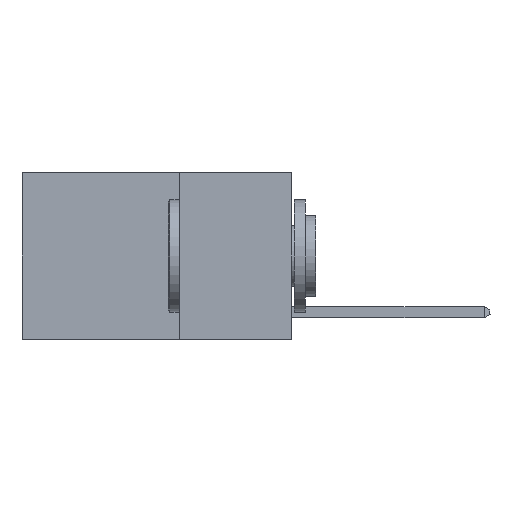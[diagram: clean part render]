
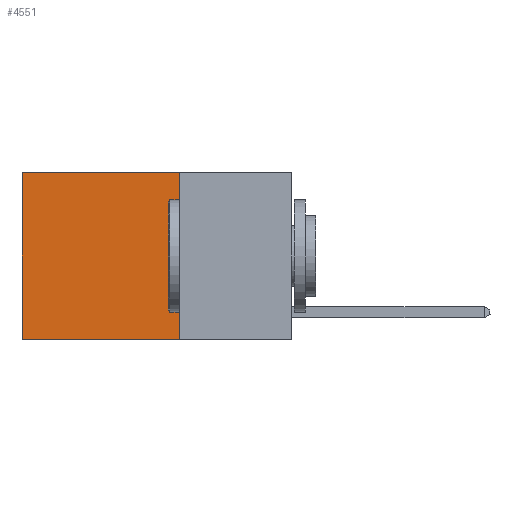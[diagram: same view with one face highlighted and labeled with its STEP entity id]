
A CAD part, left-side view. The second image highlights one B-rep face of the part: STEP entity #4551.
In plain terms, the highlighted planar face has unit normal (-1, 0, 0).
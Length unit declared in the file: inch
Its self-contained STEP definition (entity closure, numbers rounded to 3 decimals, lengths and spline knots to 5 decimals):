
#149 = LINE ( 'NONE', #9764, #9037 ) ;
#682 = CARTESIAN_POINT ( 'NONE',  ( 0.2625, 0.25, 0. ) ) ;
#2425 = CARTESIAN_POINT ( 'NONE',  ( 0.2625, 0.25, 0. ) ) ;
#2470 = DIRECTION ( 'NONE',  ( 0., 1., 0. ) ) ;
#2547 = VERTEX_POINT ( 'NONE', #7245 ) ;
#3238 = DIRECTION ( 'NONE',  ( 0., 0., -1. ) ) ;
#3993 = ORIENTED_EDGE ( 'NONE', *, *, #22213, .F. ) ;
#4204 = DIRECTION ( 'NONE',  ( 0., 0., -1. ) ) ;
#4551 = ADVANCED_FACE ( 'NONE', ( #8181 ), #9469, .F. ) ;
#6572 = EDGE_LOOP ( 'NONE', ( #8663, #3993, #18216, #15621 ) ) ;
#7245 = CARTESIAN_POINT ( 'NONE',  ( 0.2625, 0.6, -0.37 ) ) ;
#7411 = LINE ( 'NONE', #682, #20878 ) ;
#7981 = DIRECTION ( 'NONE',  ( 0., 1., 0. ) ) ;
#8181 = FACE_OUTER_BOUND ( 'NONE', #6572, .T. ) ;
#8663 = ORIENTED_EDGE ( 'NONE', *, *, #14567, .T. ) ;
#9037 = VECTOR ( 'NONE', #7981, 39.37008 ) ;
#9449 = VERTEX_POINT ( 'NONE', #22860 ) ;
#9469 = PLANE ( 'NONE',  #9526 ) ;
#9526 = AXIS2_PLACEMENT_3D ( 'NONE', #2425, #14747, #4204 ) ;
#9764 = CARTESIAN_POINT ( 'NONE',  ( 0.2625, 0.25, -0.37 ) ) ;
#9981 = VERTEX_POINT ( 'NONE', #20740 ) ;
#12970 = VECTOR ( 'NONE', #3238, 39.37008 ) ;
#13162 = CARTESIAN_POINT ( 'NONE',  ( 0.2625, 0.6, 0. ) ) ;
#13240 = EDGE_CURVE ( 'NONE', #9981, #15704, #7411, .T. ) ;
#14567 = EDGE_CURVE ( 'NONE', #15704, #2547, #15564, .T. ) ;
#14747 = DIRECTION ( 'NONE',  ( 1., 0., 0. ) ) ;
#14886 = DIRECTION ( 'NONE',  ( 0., 0., -1. ) ) ;
#15564 = LINE ( 'NONE', #13162, #16122 ) ;
#15621 = ORIENTED_EDGE ( 'NONE', *, *, #13240, .T. ) ;
#15704 = VERTEX_POINT ( 'NONE', #18037 ) ;
#16122 = VECTOR ( 'NONE', #14886, 39.37008 ) ;
#17260 = CARTESIAN_POINT ( 'NONE',  ( 0.2625, 0.25, 0. ) ) ;
#17620 = LINE ( 'NONE', #17260, #12970 ) ;
#17927 = EDGE_CURVE ( 'NONE', #9981, #9449, #17620, .T. ) ;
#18037 = CARTESIAN_POINT ( 'NONE',  ( 0.2625, 0.6, 0. ) ) ;
#18216 = ORIENTED_EDGE ( 'NONE', *, *, #17927, .F. ) ;
#20740 = CARTESIAN_POINT ( 'NONE',  ( 0.2625, 0.25, 0. ) ) ;
#20878 = VECTOR ( 'NONE', #2470, 39.37008 ) ;
#22213 = EDGE_CURVE ( 'NONE', #9449, #2547, #149, .T. ) ;
#22860 = CARTESIAN_POINT ( 'NONE',  ( 0.2625, 0.25, -0.37 ) ) ;
